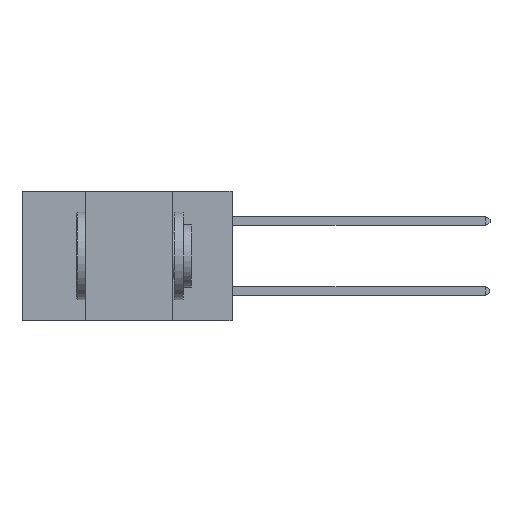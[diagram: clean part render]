
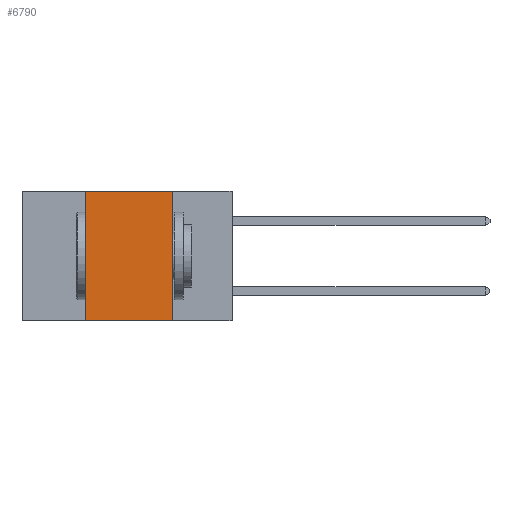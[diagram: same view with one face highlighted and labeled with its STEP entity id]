
A CAD part, left-side view. The second image highlights one B-rep face of the part: STEP entity #6790.
In plain terms, the highlighted planar face has unit normal (-1, 0, 0).
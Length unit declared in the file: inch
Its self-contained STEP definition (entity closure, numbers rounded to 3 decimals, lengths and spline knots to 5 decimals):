
#29 = ORIENTED_EDGE ( 'NONE', *, *, #2768, .F. ) ;
#90 = VECTOR ( 'NONE', #8400, 39.37008 ) ;
#175 = CARTESIAN_POINT ( 'NONE',  ( 0., 0.17, 0. ) ) ;
#332 = AXIS2_PLACEMENT_3D ( 'NONE', #6819, #7527, #3201 ) ;
#1550 = DIRECTION ( 'NONE',  ( 0., 0., -1. ) ) ;
#1642 = CARTESIAN_POINT ( 'NONE',  ( 0., 0.17, 0. ) ) ;
#2119 = VERTEX_POINT ( 'NONE', #4823 ) ;
#2179 = LINE ( 'NONE', #8415, #90 ) ;
#2282 = CARTESIAN_POINT ( 'NONE',  ( 0., 0.42, 0. ) ) ;
#2358 = ORIENTED_EDGE ( 'NONE', *, *, #5031, .F. ) ;
#2750 = LINE ( 'NONE', #6791, #4703 ) ;
#2768 = EDGE_CURVE ( 'NONE', #6922, #7832, #2179, .T. ) ;
#3201 = DIRECTION ( 'NONE',  ( 0., 0., -1. ) ) ;
#3335 = CARTESIAN_POINT ( 'NONE',  ( 0., 0.42, -0.37 ) ) ;
#3928 = EDGE_CURVE ( 'NONE', #6922, #2119, #2750, .T. ) ;
#4703 = VECTOR ( 'NONE', #6596, 39.37008 ) ;
#4823 = CARTESIAN_POINT ( 'NONE',  ( 0., 0.17, -0.37 ) ) ;
#5031 = EDGE_CURVE ( 'NONE', #8698, #2119, #5243, .T. ) ;
#5164 = CARTESIAN_POINT ( 'NONE',  ( 0., 0.6, 0. ) ) ;
#5243 = LINE ( 'NONE', #1642, #9040 ) ;
#5325 = ORIENTED_EDGE ( 'NONE', *, *, #7246, .F. ) ;
#5593 = EDGE_LOOP ( 'NONE', ( #2358, #5325, #29, #8332 ) ) ;
#6088 = PLANE ( 'NONE',  #332 ) ;
#6131 = VECTOR ( 'NONE', #9447, 39.37008 ) ;
#6369 = FACE_OUTER_BOUND ( 'NONE', #5593, .T. ) ;
#6596 = DIRECTION ( 'NONE',  ( 0., -1., 0. ) ) ;
#6790 = ADVANCED_FACE ( 'NONE', ( #6369 ), #6088, .F. ) ;
#6791 = CARTESIAN_POINT ( 'NONE',  ( 0., 0.6, -0.37 ) ) ;
#6819 = CARTESIAN_POINT ( 'NONE',  ( 0., 0.6, 0. ) ) ;
#6922 = VERTEX_POINT ( 'NONE', #3335 ) ;
#7246 = EDGE_CURVE ( 'NONE', #7832, #8698, #8021, .T. ) ;
#7527 = DIRECTION ( 'NONE',  ( 1., 0., 0. ) ) ;
#7832 = VERTEX_POINT ( 'NONE', #2282 ) ;
#8021 = LINE ( 'NONE', #5164, #6131 ) ;
#8332 = ORIENTED_EDGE ( 'NONE', *, *, #3928, .T. ) ;
#8400 = DIRECTION ( 'NONE',  ( 0., 0., 1. ) ) ;
#8415 = CARTESIAN_POINT ( 'NONE',  ( 0., 0.42, 0. ) ) ;
#8698 = VERTEX_POINT ( 'NONE', #175 ) ;
#9040 = VECTOR ( 'NONE', #1550, 39.37008 ) ;
#9447 = DIRECTION ( 'NONE',  ( 0., -1., 0. ) ) ;
